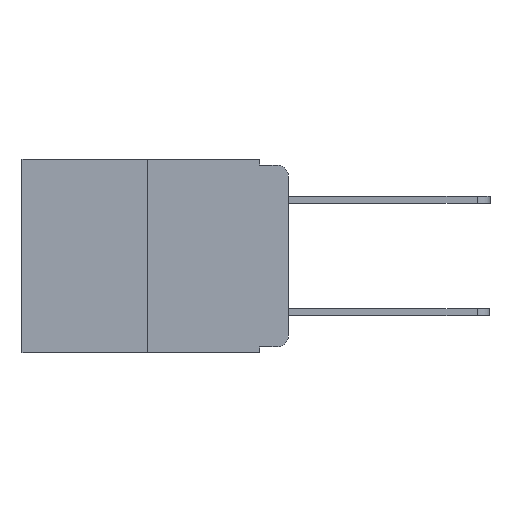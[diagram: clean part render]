
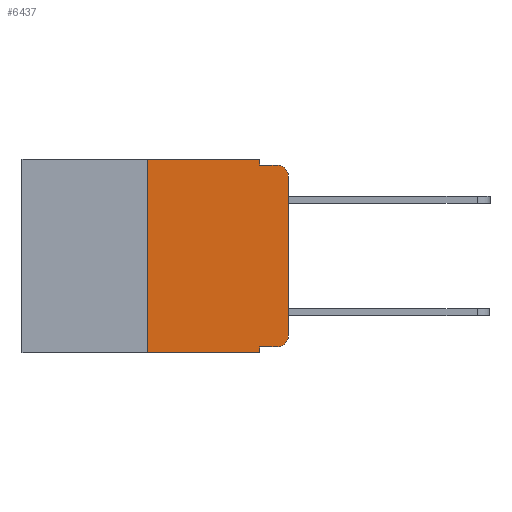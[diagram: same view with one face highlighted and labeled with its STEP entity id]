
A CAD part, left-side view. The second image highlights one B-rep face of the part: STEP entity #6437.
In plain terms, the highlighted planar face has unit normal (-1, 0, 0).
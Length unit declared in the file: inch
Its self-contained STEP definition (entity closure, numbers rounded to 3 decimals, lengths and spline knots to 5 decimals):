
#34 = LINE ( 'NONE', #14558, #18778 ) ;
#185 = EDGE_CURVE ( 'NONE', #22158, #9649, #11165, .T. ) ;
#318 = CIRCLE ( 'NONE', #22367, 0.02 ) ;
#1149 = CARTESIAN_POINT ( 'NONE',  ( 0., 0.25, 0. ) ) ;
#1154 = FACE_OUTER_BOUND ( 'NONE', #16684, .T. ) ;
#1462 = DIRECTION ( 'NONE',  ( 0., -1., 0. ) ) ;
#1670 = ORIENTED_EDGE ( 'NONE', *, *, #4534, .F. ) ;
#1894 = CARTESIAN_POINT ( 'NONE',  ( 0., 0., -0.03 ) ) ;
#2061 = VECTOR ( 'NONE', #15770, 39.37008 ) ;
#2381 = VERTEX_POINT ( 'NONE', #13699 ) ;
#2383 = CARTESIAN_POINT ( 'NONE',  ( 0., 0.051, -0.01 ) ) ;
#2438 = VERTEX_POINT ( 'NONE', #20217 ) ;
#3562 = PLANE ( 'NONE',  #16550 ) ;
#4477 = CARTESIAN_POINT ( 'NONE',  ( 0., 0.02, -0.03 ) ) ;
#4534 = EDGE_CURVE ( 'NONE', #12561, #23200, #34, .T. ) ;
#4860 = VERTEX_POINT ( 'NONE', #2383 ) ;
#5031 = VERTEX_POINT ( 'NONE', #16279 ) ;
#5838 = EDGE_CURVE ( 'NONE', #22158, #16996, #5944, .T. ) ;
#5944 = LINE ( 'NONE', #12944, #10270 ) ;
#6338 = DIRECTION ( 'NONE',  ( 0., 0., -1. ) ) ;
#6437 = ADVANCED_FACE ( 'NONE', ( #1154 ), #3562, .F. ) ;
#6455 = CIRCLE ( 'NONE', #23321, 0.02 ) ;
#6532 = ORIENTED_EDGE ( 'NONE', *, *, #15301, .F. ) ;
#6994 = DIRECTION ( 'NONE',  ( 0., 0., 1. ) ) ;
#7325 = EDGE_CURVE ( 'NONE', #2381, #16696, #7873, .T. ) ;
#7873 = LINE ( 'NONE', #23378, #21962 ) ;
#8192 = CARTESIAN_POINT ( 'NONE',  ( 0., 0.051, 0. ) ) ;
#8422 = EDGE_CURVE ( 'NONE', #4860, #2438, #14000, .T. ) ;
#8445 = VECTOR ( 'NONE', #22883, 39.37008 ) ;
#8980 = DIRECTION ( 'NONE',  ( 0., 0., 1. ) ) ;
#9175 = CARTESIAN_POINT ( 'NONE',  ( 0., 0.473, 0. ) ) ;
#9649 = VERTEX_POINT ( 'NONE', #15800 ) ;
#9852 = LINE ( 'NONE', #14432, #19178 ) ;
#10104 = CARTESIAN_POINT ( 'NONE',  ( 0., 0.051, -0.01 ) ) ;
#10167 = VECTOR ( 'NONE', #8980, 39.37008 ) ;
#10211 = CARTESIAN_POINT ( 'NONE',  ( 0., 0.02, -0.313 ) ) ;
#10270 = VECTOR ( 'NONE', #16732, 39.37008 ) ;
#11029 = DIRECTION ( 'NONE',  ( 0., 0., -1. ) ) ;
#11165 = LINE ( 'NONE', #15626, #2061 ) ;
#11460 = ORIENTED_EDGE ( 'NONE', *, *, #16002, .T. ) ;
#12083 = DIRECTION ( 'NONE',  ( 0., 0., -1. ) ) ;
#12561 = VERTEX_POINT ( 'NONE', #1149 ) ;
#12944 = CARTESIAN_POINT ( 'NONE',  ( 0., 0.051, -0.333 ) ) ;
#13699 = CARTESIAN_POINT ( 'NONE',  ( 0., 0., -0.313 ) ) ;
#14000 = LINE ( 'NONE', #10104, #8445 ) ;
#14366 = EDGE_CURVE ( 'NONE', #16696, #2438, #6455, .T. ) ;
#14432 = CARTESIAN_POINT ( 'NONE',  ( 0., 0.473, -0.343 ) ) ;
#14558 = CARTESIAN_POINT ( 'NONE',  ( 0., 0.473, 0. ) ) ;
#14818 = VECTOR ( 'NONE', #19347, 39.37008 ) ;
#15301 = EDGE_CURVE ( 'NONE', #5031, #12561, #20559, .T. ) ;
#15626 = CARTESIAN_POINT ( 'NONE',  ( 0., 0.051, 0. ) ) ;
#15770 = DIRECTION ( 'NONE',  ( 0., 0., -1. ) ) ;
#15783 = ORIENTED_EDGE ( 'NONE', *, *, #7325, .T. ) ;
#15800 = CARTESIAN_POINT ( 'NONE',  ( 0., 0.051, -0.343 ) ) ;
#15883 = ORIENTED_EDGE ( 'NONE', *, *, #14366, .T. ) ;
#15930 = ORIENTED_EDGE ( 'NONE', *, *, #8422, .F. ) ;
#16002 = EDGE_CURVE ( 'NONE', #5031, #9649, #9852, .T. ) ;
#16279 = CARTESIAN_POINT ( 'NONE',  ( 0., 0.25, -0.343 ) ) ;
#16433 = CARTESIAN_POINT ( 'NONE',  ( 0., 0.25, 0. ) ) ;
#16441 = EDGE_CURVE ( 'NONE', #23200, #4860, #19695, .T. ) ;
#16550 = AXIS2_PLACEMENT_3D ( 'NONE', #9175, #21996, #11029 ) ;
#16684 = EDGE_LOOP ( 'NONE', ( #15783, #15883, #15930, #16795, #1670, #6532, #11460, #21802, #16787, #22083 ) ) ;
#16696 = VERTEX_POINT ( 'NONE', #1894 ) ;
#16732 = DIRECTION ( 'NONE',  ( 0., -1., 0. ) ) ;
#16787 = ORIENTED_EDGE ( 'NONE', *, *, #5838, .T. ) ;
#16795 = ORIENTED_EDGE ( 'NONE', *, *, #16441, .F. ) ;
#16996 = VERTEX_POINT ( 'NONE', #22969 ) ;
#17509 = DIRECTION ( 'NONE',  ( -1., 0., 0. ) ) ;
#18254 = EDGE_CURVE ( 'NONE', #16996, #2381, #318, .T. ) ;
#18674 = CARTESIAN_POINT ( 'NONE',  ( 0., 0.051, -0.333 ) ) ;
#18778 = VECTOR ( 'NONE', #1462, 39.37008 ) ;
#19178 = VECTOR ( 'NONE', #23387, 39.37008 ) ;
#19347 = DIRECTION ( 'NONE',  ( 0., 0., -1. ) ) ;
#19695 = LINE ( 'NONE', #8192, #14818 ) ;
#20167 = CARTESIAN_POINT ( 'NONE',  ( 0., 0.051, 0. ) ) ;
#20217 = CARTESIAN_POINT ( 'NONE',  ( 0., 0.02, -0.01 ) ) ;
#20559 = LINE ( 'NONE', #16433, #10167 ) ;
#21802 = ORIENTED_EDGE ( 'NONE', *, *, #185, .F. ) ;
#21962 = VECTOR ( 'NONE', #6994, 39.37008 ) ;
#21996 = DIRECTION ( 'NONE',  ( 1., 0., 0. ) ) ;
#22083 = ORIENTED_EDGE ( 'NONE', *, *, #18254, .T. ) ;
#22158 = VERTEX_POINT ( 'NONE', #18674 ) ;
#22367 = AXIS2_PLACEMENT_3D ( 'NONE', #10211, #22988, #12083 ) ;
#22883 = DIRECTION ( 'NONE',  ( 0., -1., 0. ) ) ;
#22969 = CARTESIAN_POINT ( 'NONE',  ( 0., 0.02, -0.333 ) ) ;
#22988 = DIRECTION ( 'NONE',  ( -1., 0., 0. ) ) ;
#23200 = VERTEX_POINT ( 'NONE', #20167 ) ;
#23321 = AXIS2_PLACEMENT_3D ( 'NONE', #4477, #17509, #6338 ) ;
#23378 = CARTESIAN_POINT ( 'NONE',  ( 0., 0., 0. ) ) ;
#23387 = DIRECTION ( 'NONE',  ( 0., -1., 0. ) ) ;
